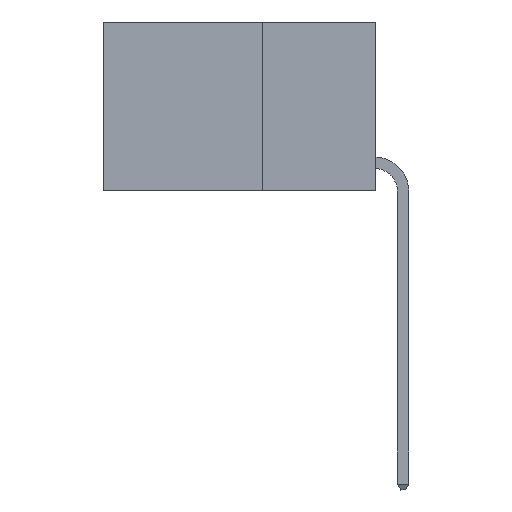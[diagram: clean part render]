
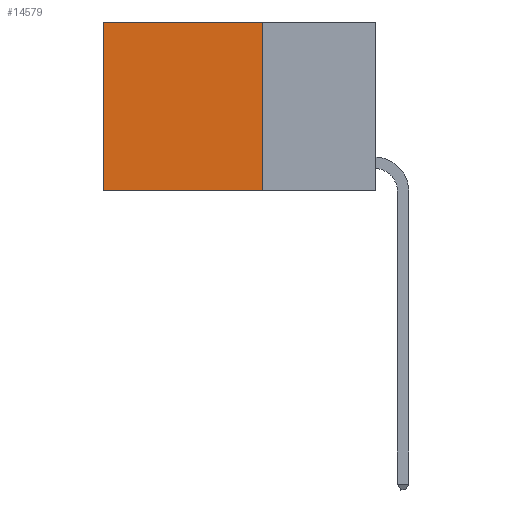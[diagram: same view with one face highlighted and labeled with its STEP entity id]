
A CAD part, left-side view. The second image highlights one B-rep face of the part: STEP entity #14579.
In plain terms, the highlighted planar face has unit normal (-1, 0, 0).
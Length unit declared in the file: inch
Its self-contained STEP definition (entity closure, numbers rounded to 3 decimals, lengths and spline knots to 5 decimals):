
#100 = DIRECTION ( 'NONE',  ( 0., 0., -1. ) ) ;
#2244 = VERTEX_POINT ( 'NONE', #7264 ) ;
#2675 = CARTESIAN_POINT ( 'NONE',  ( 0.2625, 0.25, 0. ) ) ;
#3393 = VECTOR ( 'NONE', #15876, 39.37008 ) ;
#3842 = VERTEX_POINT ( 'NONE', #11840 ) ;
#4352 = LINE ( 'NONE', #6733, #15225 ) ;
#4493 = VECTOR ( 'NONE', #13026, 39.37008 ) ;
#4938 = VECTOR ( 'NONE', #7030, 39.37008 ) ;
#4978 = ORIENTED_EDGE ( 'NONE', *, *, #12425, .T. ) ;
#5041 = EDGE_CURVE ( 'NONE', #3842, #12330, #15646, .T. ) ;
#5519 = DIRECTION ( 'NONE',  ( 0., 1., 0. ) ) ;
#5654 = LINE ( 'NONE', #15583, #4493 ) ;
#5918 = EDGE_CURVE ( 'NONE', #3842, #2244, #4352, .T. ) ;
#6397 = DIRECTION ( 'NONE',  ( 1., 0., 0. ) ) ;
#6733 = CARTESIAN_POINT ( 'NONE',  ( 0.2625, 0.25, 0. ) ) ;
#7030 = DIRECTION ( 'NONE',  ( 0., 0., -1. ) ) ;
#7264 = CARTESIAN_POINT ( 'NONE',  ( 0.2625, 0.6, 0. ) ) ;
#7905 = VERTEX_POINT ( 'NONE', #9016 ) ;
#8352 = ORIENTED_EDGE ( 'NONE', *, *, #5918, .T. ) ;
#8671 = EDGE_LOOP ( 'NONE', ( #4978, #11623, #15984, #8352 ) ) ;
#8694 = AXIS2_PLACEMENT_3D ( 'NONE', #2675, #6397, #100 ) ;
#9016 = CARTESIAN_POINT ( 'NONE',  ( 0.2625, 0.6, -0.37 ) ) ;
#11623 = ORIENTED_EDGE ( 'NONE', *, *, #13429, .F. ) ;
#11840 = CARTESIAN_POINT ( 'NONE',  ( 0.2625, 0.25, 0. ) ) ;
#12330 = VERTEX_POINT ( 'NONE', #15203 ) ;
#12425 = EDGE_CURVE ( 'NONE', #2244, #7905, #14459, .T. ) ;
#12699 = PLANE ( 'NONE',  #8694 ) ;
#13026 = DIRECTION ( 'NONE',  ( 0., 1., 0. ) ) ;
#13248 = CARTESIAN_POINT ( 'NONE',  ( 0.2625, 0.25, 0. ) ) ;
#13429 = EDGE_CURVE ( 'NONE', #12330, #7905, #5654, .T. ) ;
#14079 = FACE_OUTER_BOUND ( 'NONE', #8671, .T. ) ;
#14459 = LINE ( 'NONE', #14624, #3393 ) ;
#14579 = ADVANCED_FACE ( 'NONE', ( #14079 ), #12699, .F. ) ;
#14624 = CARTESIAN_POINT ( 'NONE',  ( 0.2625, 0.6, 0. ) ) ;
#15203 = CARTESIAN_POINT ( 'NONE',  ( 0.2625, 0.25, -0.37 ) ) ;
#15225 = VECTOR ( 'NONE', #5519, 39.37008 ) ;
#15583 = CARTESIAN_POINT ( 'NONE',  ( 0.2625, 0.25, -0.37 ) ) ;
#15646 = LINE ( 'NONE', #13248, #4938 ) ;
#15876 = DIRECTION ( 'NONE',  ( 0., 0., -1. ) ) ;
#15984 = ORIENTED_EDGE ( 'NONE', *, *, #5041, .F. ) ;
